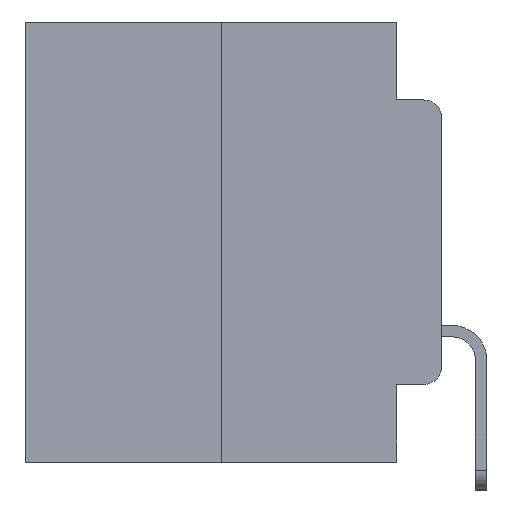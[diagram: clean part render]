
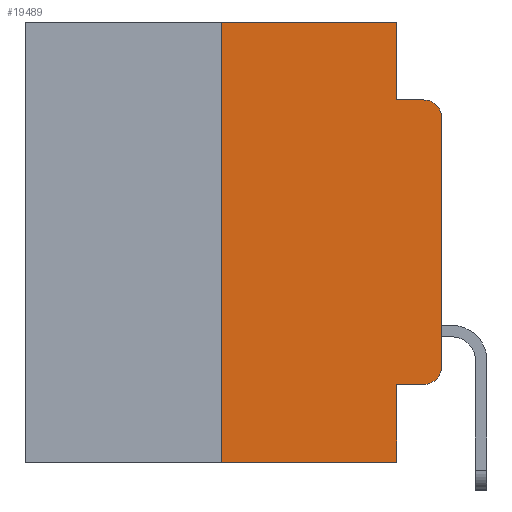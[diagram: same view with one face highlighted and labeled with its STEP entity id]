
A CAD part, left-side view. The second image highlights one B-rep face of the part: STEP entity #19489.
In plain terms, the highlighted planar face has unit normal (-1, 0, 0).
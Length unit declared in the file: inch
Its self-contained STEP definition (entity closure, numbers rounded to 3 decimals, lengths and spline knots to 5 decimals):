
#413 = LINE ( 'NONE', #14477, #5366 ) ;
#872 = CARTESIAN_POINT ( 'NONE',  ( 0., 0.051, -0.4115 ) ) ;
#1401 = CARTESIAN_POINT ( 'NONE',  ( 0., 0.473, 0. ) ) ;
#1617 = ORIENTED_EDGE ( 'NONE', *, *, #10597, .F. ) ;
#1768 = VECTOR ( 'NONE', #20686, 39.37008 ) ;
#2092 = ORIENTED_EDGE ( 'NONE', *, *, #9203, .F. ) ;
#2489 = VERTEX_POINT ( 'NONE', #10771 ) ;
#2761 = LINE ( 'NONE', #4551, #8319 ) ;
#3018 = ORIENTED_EDGE ( 'NONE', *, *, #19936, .F. ) ;
#3263 = ORIENTED_EDGE ( 'NONE', *, *, #7852, .F. ) ;
#3647 = DIRECTION ( 'NONE',  ( 0., 0., -1. ) ) ;
#3667 = EDGE_CURVE ( 'NONE', #2489, #15742, #14832, .T. ) ;
#3901 = CARTESIAN_POINT ( 'NONE',  ( 0., 0.25, 0. ) ) ;
#4257 = VECTOR ( 'NONE', #3647, 39.37008 ) ;
#4261 = ORIENTED_EDGE ( 'NONE', *, *, #19698, .T. ) ;
#4419 = LINE ( 'NONE', #19239, #14697 ) ;
#4545 = DIRECTION ( 'NONE',  ( 0., -1., 0. ) ) ;
#4551 = CARTESIAN_POINT ( 'NONE',  ( 0., 0.473, -0.5 ) ) ;
#4909 = ORIENTED_EDGE ( 'NONE', *, *, #6476, .F. ) ;
#5085 = EDGE_CURVE ( 'NONE', #23825, #2489, #15700, .T. ) ;
#5278 = AXIS2_PLACEMENT_3D ( 'NONE', #24764, #24795, #24626 ) ;
#5366 = VECTOR ( 'NONE', #24625, 39.37008 ) ;
#5648 = PLANE ( 'NONE',  #18120 ) ;
#5774 = VERTEX_POINT ( 'NONE', #20230 ) ;
#5956 = CARTESIAN_POINT ( 'NONE',  ( 0., 0.02, -0.0885 ) ) ;
#6204 = ORIENTED_EDGE ( 'NONE', *, *, #5085, .T. ) ;
#6323 = CARTESIAN_POINT ( 'NONE',  ( 0., 0.473, 0. ) ) ;
#6476 = EDGE_CURVE ( 'NONE', #23825, #16782, #413, .T. ) ;
#6694 = VERTEX_POINT ( 'NONE', #19205 ) ;
#6921 = DIRECTION ( 'NONE',  ( 0., -1., 0. ) ) ;
#7715 = DIRECTION ( 'NONE',  ( 0., 0., -1. ) ) ;
#7852 = EDGE_CURVE ( 'NONE', #5774, #20395, #23554, .T. ) ;
#7870 = VECTOR ( 'NONE', #18267, 39.37008 ) ;
#8319 = VECTOR ( 'NONE', #18901, 39.37008 ) ;
#8809 = CARTESIAN_POINT ( 'NONE',  ( 0., 0., -0.3915 ) ) ;
#9022 = VECTOR ( 'NONE', #6921, 39.37008 ) ;
#9203 = EDGE_CURVE ( 'NONE', #24057, #6694, #20643, .T. ) ;
#9274 = DIRECTION ( 'NONE',  ( -1., 0., 0. ) ) ;
#10597 = EDGE_CURVE ( 'NONE', #6694, #17011, #25286, .T. ) ;
#10771 = CARTESIAN_POINT ( 'NONE',  ( 0., 0.02, -0.4115 ) ) ;
#11073 = DIRECTION ( 'NONE',  ( 0., 0., 1. ) ) ;
#11199 = FACE_OUTER_BOUND ( 'NONE', #25338, .T. ) ;
#11210 = AXIS2_PLACEMENT_3D ( 'NONE', #21599, #9274, #23600 ) ;
#11942 = EDGE_CURVE ( 'NONE', #23303, #17011, #24980, .T. ) ;
#13216 = ORIENTED_EDGE ( 'NONE', *, *, #11942, .T. ) ;
#13283 = CARTESIAN_POINT ( 'NONE',  ( 0., 0.051, -0.4115 ) ) ;
#13354 = EDGE_CURVE ( 'NONE', #15742, #23303, #4419, .T. ) ;
#13932 = CARTESIAN_POINT ( 'NONE',  ( 0., 0.051, 0. ) ) ;
#14109 = CARTESIAN_POINT ( 'NONE',  ( 0., 0., -0.1085 ) ) ;
#14477 = CARTESIAN_POINT ( 'NONE',  ( 0., 0.051, 0. ) ) ;
#14697 = VECTOR ( 'NONE', #11073, 39.37008 ) ;
#14832 = CIRCLE ( 'NONE', #5278, 0.02 ) ;
#15700 = LINE ( 'NONE', #13283, #25864 ) ;
#15742 = VERTEX_POINT ( 'NONE', #8809 ) ;
#16782 = VERTEX_POINT ( 'NONE', #25499 ) ;
#17011 = VERTEX_POINT ( 'NONE', #5956 ) ;
#18120 = AXIS2_PLACEMENT_3D ( 'NONE', #1401, #19991, #7715 ) ;
#18267 = DIRECTION ( 'NONE',  ( 0., 0., 1. ) ) ;
#18901 = DIRECTION ( 'NONE',  ( 0., -1., 0. ) ) ;
#19205 = CARTESIAN_POINT ( 'NONE',  ( 0., 0.051, -0.0885 ) ) ;
#19239 = CARTESIAN_POINT ( 'NONE',  ( 0., 0., 0. ) ) ;
#19489 = ADVANCED_FACE ( 'NONE', ( #11199 ), #5648, .F. ) ;
#19698 = EDGE_CURVE ( 'NONE', #5774, #16782, #2761, .T. ) ;
#19936 = EDGE_CURVE ( 'NONE', #20395, #24057, #21785, .T. ) ;
#19970 = ORIENTED_EDGE ( 'NONE', *, *, #3667, .T. ) ;
#19991 = DIRECTION ( 'NONE',  ( 1., 0., 0. ) ) ;
#20230 = CARTESIAN_POINT ( 'NONE',  ( 0., 0.25, -0.5 ) ) ;
#20395 = VERTEX_POINT ( 'NONE', #20467 ) ;
#20467 = CARTESIAN_POINT ( 'NONE',  ( 0., 0.25, 0. ) ) ;
#20643 = LINE ( 'NONE', #13932, #4257 ) ;
#20686 = DIRECTION ( 'NONE',  ( 0., -1., 0. ) ) ;
#21599 = CARTESIAN_POINT ( 'NONE',  ( 0., 0.02, -0.1085 ) ) ;
#21785 = LINE ( 'NONE', #6323, #1768 ) ;
#23230 = CARTESIAN_POINT ( 'NONE',  ( 0., 0.051, -0.0885 ) ) ;
#23303 = VERTEX_POINT ( 'NONE', #14109 ) ;
#23421 = ORIENTED_EDGE ( 'NONE', *, *, #13354, .T. ) ;
#23554 = LINE ( 'NONE', #3901, #7870 ) ;
#23600 = DIRECTION ( 'NONE',  ( 0., 0., -1. ) ) ;
#23825 = VERTEX_POINT ( 'NONE', #872 ) ;
#24057 = VERTEX_POINT ( 'NONE', #24144 ) ;
#24144 = CARTESIAN_POINT ( 'NONE',  ( 0., 0.051, 0. ) ) ;
#24625 = DIRECTION ( 'NONE',  ( 0., 0., -1. ) ) ;
#24626 = DIRECTION ( 'NONE',  ( 0., 0., -1. ) ) ;
#24764 = CARTESIAN_POINT ( 'NONE',  ( 0., 0.02, -0.3915 ) ) ;
#24795 = DIRECTION ( 'NONE',  ( -1., 0., 0. ) ) ;
#24980 = CIRCLE ( 'NONE', #11210, 0.02 ) ;
#25286 = LINE ( 'NONE', #23230, #9022 ) ;
#25338 = EDGE_LOOP ( 'NONE', ( #23421, #13216, #1617, #2092, #3018, #3263, #4261, #4909, #6204, #19970 ) ) ;
#25499 = CARTESIAN_POINT ( 'NONE',  ( 0., 0.051, -0.5 ) ) ;
#25864 = VECTOR ( 'NONE', #4545, 39.37008 ) ;
